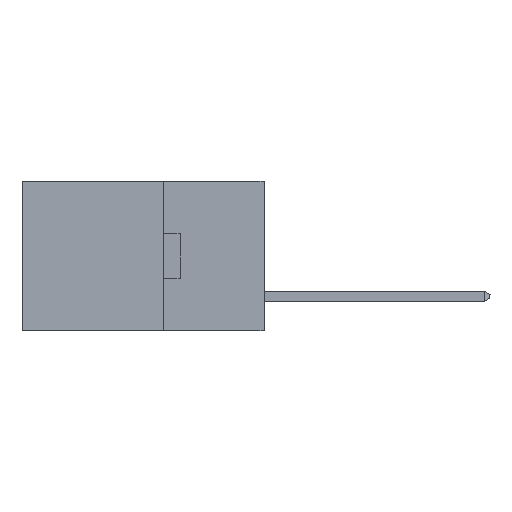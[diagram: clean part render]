
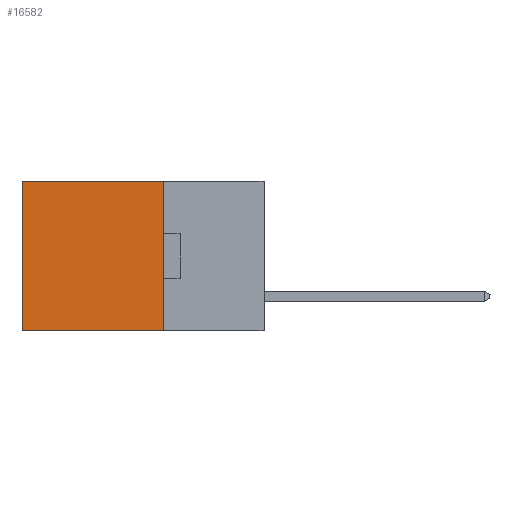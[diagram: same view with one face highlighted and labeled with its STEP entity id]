
A CAD part, left-side view. The second image highlights one B-rep face of the part: STEP entity #16582.
In plain terms, the highlighted planar face has unit normal (-1, 0, 0).
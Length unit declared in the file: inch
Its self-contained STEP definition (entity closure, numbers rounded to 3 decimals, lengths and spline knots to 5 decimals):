
#1009 = VERTEX_POINT ( 'NONE', #14544 ) ;
#1668 = CARTESIAN_POINT ( 'NONE',  ( 0.2615, 0.6, 0. ) ) ;
#2354 = CARTESIAN_POINT ( 'NONE',  ( 0.2615, 0.25, 0. ) ) ;
#2381 = VECTOR ( 'NONE', #25626, 39.37008 ) ;
#2477 = EDGE_CURVE ( 'NONE', #1009, #15778, #4983, .T. ) ;
#2702 = VECTOR ( 'NONE', #25457, 39.37008 ) ;
#3464 = ORIENTED_EDGE ( 'NONE', *, *, #2477, .T. ) ;
#4983 = LINE ( 'NONE', #2354, #2381 ) ;
#5498 = VECTOR ( 'NONE', #21840, 39.37008 ) ;
#7559 = CARTESIAN_POINT ( 'NONE',  ( 0.2615, 0.25, -0.37 ) ) ;
#7824 = VECTOR ( 'NONE', #21456, 39.37008 ) ;
#7831 = DIRECTION ( 'NONE',  ( 1., 0., 0. ) ) ;
#7842 = CARTESIAN_POINT ( 'NONE',  ( 0.2615, 0.25, -0.37 ) ) ;
#8401 = EDGE_CURVE ( 'NONE', #14685, #11823, #25738, .T. ) ;
#8710 = LINE ( 'NONE', #10918, #7824 ) ;
#9930 = CARTESIAN_POINT ( 'NONE',  ( 0.2615, 0.6, -0.37 ) ) ;
#10268 = EDGE_CURVE ( 'NONE', #1009, #14685, #11450, .T. ) ;
#10918 = CARTESIAN_POINT ( 'NONE',  ( 0.2615, 0.6, -0.37 ) ) ;
#11450 = LINE ( 'NONE', #7559, #5498 ) ;
#11823 = VERTEX_POINT ( 'NONE', #9930 ) ;
#13372 = ORIENTED_EDGE ( 'NONE', *, *, #17104, .T. ) ;
#14193 = CARTESIAN_POINT ( 'NONE',  ( 0.2615, 0.25, -0.37 ) ) ;
#14544 = CARTESIAN_POINT ( 'NONE',  ( 0.2615, 0.25, 0. ) ) ;
#14685 = VERTEX_POINT ( 'NONE', #7842 ) ;
#15778 = VERTEX_POINT ( 'NONE', #1668 ) ;
#16582 = ADVANCED_FACE ( 'NONE', ( #17038 ), #21081, .F. ) ;
#16991 = CARTESIAN_POINT ( 'NONE',  ( 0.2615, 0.25, -0.37 ) ) ;
#17038 = FACE_OUTER_BOUND ( 'NONE', #17789, .T. ) ;
#17104 = EDGE_CURVE ( 'NONE', #15778, #11823, #8710, .T. ) ;
#17789 = EDGE_LOOP ( 'NONE', ( #13372, #21889, #21544, #3464 ) ) ;
#21081 = PLANE ( 'NONE',  #22855 ) ;
#21456 = DIRECTION ( 'NONE',  ( 0., 0., -1. ) ) ;
#21544 = ORIENTED_EDGE ( 'NONE', *, *, #10268, .F. ) ;
#21840 = DIRECTION ( 'NONE',  ( 0., 0., -1. ) ) ;
#21889 = ORIENTED_EDGE ( 'NONE', *, *, #8401, .F. ) ;
#22855 = AXIS2_PLACEMENT_3D ( 'NONE', #14193, #7831, #23154 ) ;
#23154 = DIRECTION ( 'NONE',  ( 0., 0., -1. ) ) ;
#25457 = DIRECTION ( 'NONE',  ( 0., 1., 0. ) ) ;
#25626 = DIRECTION ( 'NONE',  ( 0., 1., 0. ) ) ;
#25738 = LINE ( 'NONE', #16991, #2702 ) ;
